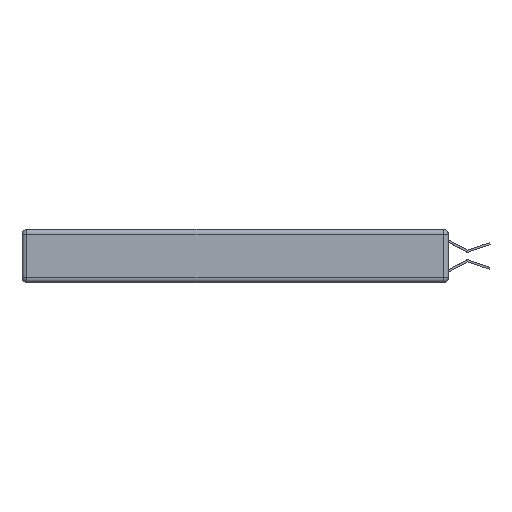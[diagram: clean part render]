
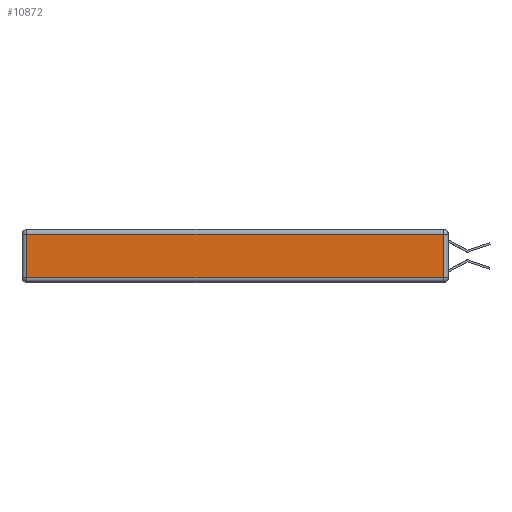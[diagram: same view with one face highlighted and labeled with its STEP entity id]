
A CAD part, left-side view. The second image highlights one B-rep face of the part: STEP entity #10872.
In plain terms, the highlighted planar face has unit normal (-1, 0, 0).
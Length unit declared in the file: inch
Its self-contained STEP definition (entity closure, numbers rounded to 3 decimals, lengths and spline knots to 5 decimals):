
#203 = VECTOR ( 'NONE', #8097, 39.37008 ) ;
#491 = CARTESIAN_POINT ( 'NONE',  ( 0., 0., -0.343 ) ) ;
#548 = PLANE ( 'NONE',  #10921 ) ;
#1625 = CARTESIAN_POINT ( 'NONE',  ( 0., 0.03, -0.343 ) ) ;
#3364 = EDGE_CURVE ( 'NONE', #10699, #16382, #4320, .T. ) ;
#3417 = CARTESIAN_POINT ( 'NONE',  ( 0., 0., -0.313 ) ) ;
#4185 = VECTOR ( 'NONE', #13832, 39.37008 ) ;
#4306 = EDGE_CURVE ( 'NONE', #10025, #10699, #16163, .T. ) ;
#4320 = LINE ( 'NONE', #13785, #203 ) ;
#4523 = VECTOR ( 'NONE', #18114, 39.37008 ) ;
#4663 = DIRECTION ( 'NONE',  ( 0., 1., 0. ) ) ;
#5551 = VERTEX_POINT ( 'NONE', #14106 ) ;
#5644 = ORIENTED_EDGE ( 'NONE', *, *, #15245, .T. ) ;
#6949 = LINE ( 'NONE', #3417, #4185 ) ;
#7781 = VECTOR ( 'NONE', #4663, 39.37008 ) ;
#7791 = EDGE_CURVE ( 'NONE', #16382, #5551, #6949, .T. ) ;
#8097 = DIRECTION ( 'NONE',  ( 0., 0., -1. ) ) ;
#8722 = LINE ( 'NONE', #1625, #4523 ) ;
#9098 = FACE_OUTER_BOUND ( 'NONE', #12924, .T. ) ;
#10025 = VERTEX_POINT ( 'NONE', #10449 ) ;
#10449 = CARTESIAN_POINT ( 'NONE',  ( 0., 0.03, -0.03 ) ) ;
#10699 = VERTEX_POINT ( 'NONE', #14707 ) ;
#10872 = ADVANCED_FACE ( 'NONE', ( #9098 ), #548, .T. ) ;
#10921 = AXIS2_PLACEMENT_3D ( 'NONE', #491, #13998, #12611 ) ;
#12611 = DIRECTION ( 'NONE',  ( 0., 0., 1. ) ) ;
#12924 = EDGE_LOOP ( 'NONE', ( #17156, #5644, #15607, #16811 ) ) ;
#13752 = CARTESIAN_POINT ( 'NONE',  ( 0., 2.75, -0.03 ) ) ;
#13785 = CARTESIAN_POINT ( 'NONE',  ( 0., 2.72, -0.343 ) ) ;
#13832 = DIRECTION ( 'NONE',  ( 0., -1., 0. ) ) ;
#13998 = DIRECTION ( 'NONE',  ( -1., 0., 0. ) ) ;
#14106 = CARTESIAN_POINT ( 'NONE',  ( 0., 0.03, -0.313 ) ) ;
#14707 = CARTESIAN_POINT ( 'NONE',  ( 0., 2.72, -0.03 ) ) ;
#15245 = EDGE_CURVE ( 'NONE', #5551, #10025, #8722, .T. ) ;
#15607 = ORIENTED_EDGE ( 'NONE', *, *, #4306, .T. ) ;
#16163 = LINE ( 'NONE', #13752, #7781 ) ;
#16382 = VERTEX_POINT ( 'NONE', #17739 ) ;
#16811 = ORIENTED_EDGE ( 'NONE', *, *, #3364, .T. ) ;
#17156 = ORIENTED_EDGE ( 'NONE', *, *, #7791, .T. ) ;
#17739 = CARTESIAN_POINT ( 'NONE',  ( 0., 2.72, -0.313 ) ) ;
#18114 = DIRECTION ( 'NONE',  ( 0., 0., 1. ) ) ;
